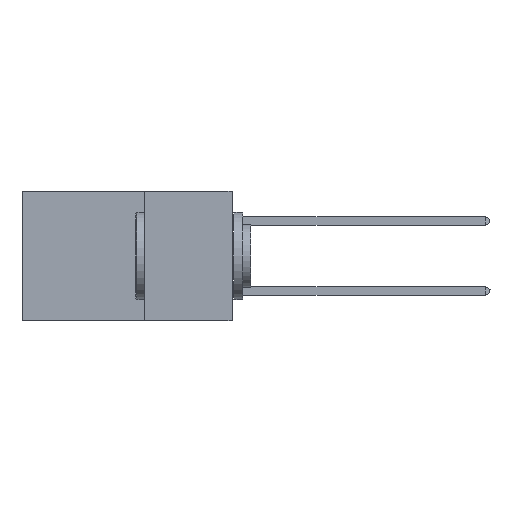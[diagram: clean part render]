
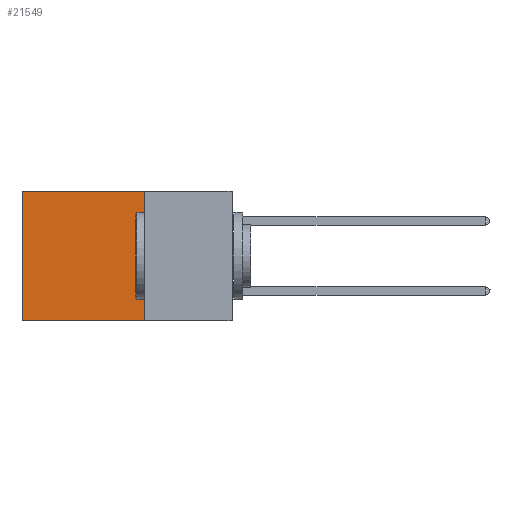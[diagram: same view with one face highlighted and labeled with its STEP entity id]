
A CAD part, left-side view. The second image highlights one B-rep face of the part: STEP entity #21549.
In plain terms, the highlighted planar face has unit normal (-1, 0, 0).
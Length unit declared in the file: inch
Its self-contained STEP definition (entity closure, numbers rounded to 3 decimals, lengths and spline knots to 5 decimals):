
#851 = DIRECTION ( 'NONE',  ( 0., 1., 0. ) ) ;
#2123 = ORIENTED_EDGE ( 'NONE', *, *, #24904, .F. ) ;
#2168 = VERTEX_POINT ( 'NONE', #17521 ) ;
#4216 = EDGE_CURVE ( 'NONE', #7439, #19125, #21983, .T. ) ;
#4633 = PLANE ( 'NONE',  #18083 ) ;
#5234 = LINE ( 'NONE', #13538, #17450 ) ;
#5299 = EDGE_LOOP ( 'NONE', ( #13235, #2123, #21518, #7904 ) ) ;
#6815 = VECTOR ( 'NONE', #9883, 39.37008 ) ;
#7439 = VERTEX_POINT ( 'NONE', #16417 ) ;
#7513 = CARTESIAN_POINT ( 'NONE',  ( 0.2875, 0.6, 0. ) ) ;
#7904 = ORIENTED_EDGE ( 'NONE', *, *, #12297, .T. ) ;
#7956 = CARTESIAN_POINT ( 'NONE',  ( 0.2875, 0.25, 0. ) ) ;
#9777 = LINE ( 'NONE', #20422, #6815 ) ;
#9883 = DIRECTION ( 'NONE',  ( 0., 0., -1. ) ) ;
#11035 = DIRECTION ( 'NONE',  ( 1., 0., 0. ) ) ;
#12297 = EDGE_CURVE ( 'NONE', #7439, #19506, #16675, .T. ) ;
#13235 = ORIENTED_EDGE ( 'NONE', *, *, #26873, .T. ) ;
#13538 = CARTESIAN_POINT ( 'NONE',  ( 0.2875, 0.25, -0.37 ) ) ;
#15175 = DIRECTION ( 'NONE',  ( 0., 1., 0. ) ) ;
#16417 = CARTESIAN_POINT ( 'NONE',  ( 0.2875, 0.25, 0. ) ) ;
#16675 = LINE ( 'NONE', #23509, #18647 ) ;
#16992 = CARTESIAN_POINT ( 'NONE',  ( 0.2875, 0.25, 0. ) ) ;
#17450 = VECTOR ( 'NONE', #851, 39.37008 ) ;
#17521 = CARTESIAN_POINT ( 'NONE',  ( 0.2875, 0.6, -0.37 ) ) ;
#18083 = AXIS2_PLACEMENT_3D ( 'NONE', #16992, #11035, #19093 ) ;
#18647 = VECTOR ( 'NONE', #15175, 39.37008 ) ;
#19093 = DIRECTION ( 'NONE',  ( 0., 0., -1. ) ) ;
#19125 = VERTEX_POINT ( 'NONE', #26466 ) ;
#19229 = FACE_OUTER_BOUND ( 'NONE', #5299, .T. ) ;
#19506 = VERTEX_POINT ( 'NONE', #7513 ) ;
#20371 = VECTOR ( 'NONE', #24375, 39.37008 ) ;
#20422 = CARTESIAN_POINT ( 'NONE',  ( 0.2875, 0.6, 0. ) ) ;
#21518 = ORIENTED_EDGE ( 'NONE', *, *, #4216, .F. ) ;
#21549 = ADVANCED_FACE ( 'NONE', ( #19229 ), #4633, .F. ) ;
#21983 = LINE ( 'NONE', #7956, #20371 ) ;
#23509 = CARTESIAN_POINT ( 'NONE',  ( 0.2875, 0.25, 0. ) ) ;
#24375 = DIRECTION ( 'NONE',  ( 0., 0., -1. ) ) ;
#24904 = EDGE_CURVE ( 'NONE', #19125, #2168, #5234, .T. ) ;
#26466 = CARTESIAN_POINT ( 'NONE',  ( 0.2875, 0.25, -0.37 ) ) ;
#26873 = EDGE_CURVE ( 'NONE', #19506, #2168, #9777, .T. ) ;
